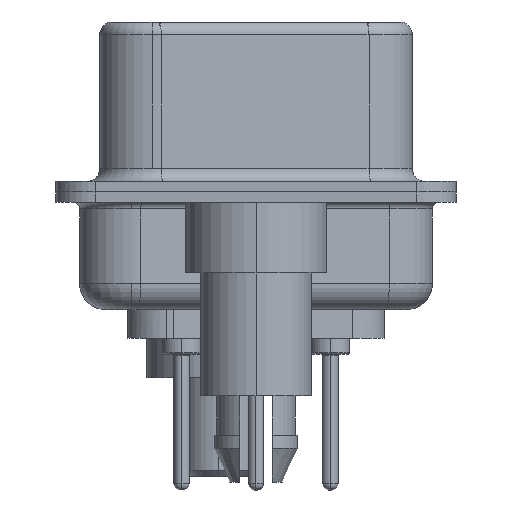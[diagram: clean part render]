
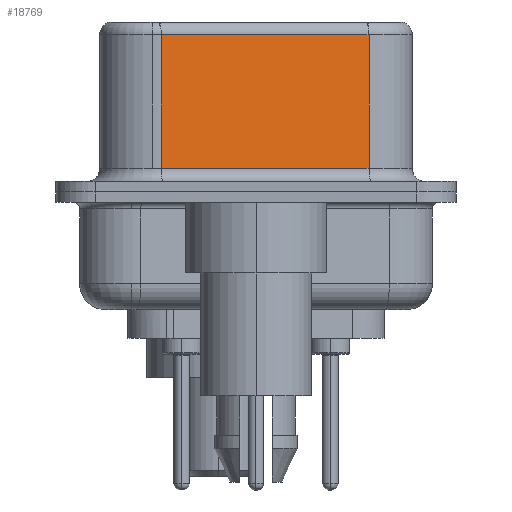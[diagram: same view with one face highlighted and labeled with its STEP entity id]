
A CAD part, left-side view. The second image highlights one B-rep face of the part: STEP entity #18769.
In plain terms, the highlighted planar face has unit normal (-0.985, -0.174, 0).
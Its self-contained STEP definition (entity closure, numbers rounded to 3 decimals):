
#282 = ORIENTED_EDGE ( 'NONE', *, *, #14902, .T. ) ;
#1563 = CARTESIAN_POINT ( 'NONE',  ( 3.73, 3.628, 6.02 ) ) ;
#2140 = VECTOR ( 'NONE', #11629, 1000. ) ;
#2462 = EDGE_CURVE ( 'NONE', #9417, #10179, #24107, .T. ) ;
#3331 = VERTEX_POINT ( 'NONE', #27265 ) ;
#6286 = ORIENTED_EDGE ( 'NONE', *, *, #25383, .T. ) ;
#7864 = CARTESIAN_POINT ( 'NONE',  ( 5.132, -4.322, 6.02 ) ) ;
#8260 = FACE_OUTER_BOUND ( 'NONE', #10070, .T. ) ;
#9417 = VERTEX_POINT ( 'NONE', #7864 ) ;
#9954 = CARTESIAN_POINT ( 'NONE',  ( 3.73, 3.628, 6.52 ) ) ;
#9983 = CARTESIAN_POINT ( 'NONE',  ( 5.132, -4.322, 6.02 ) ) ;
#10053 = CARTESIAN_POINT ( 'NONE',  ( 5.132, -4.322, 0.9 ) ) ;
#10059 = VERTEX_POINT ( 'NONE', #10053 ) ;
#10070 = EDGE_LOOP ( 'NONE', ( #21102, #13907, #282, #6286 ) ) ;
#10179 = VERTEX_POINT ( 'NONE', #1563 ) ;
#10293 = LINE ( 'NONE', #9954, #21693 ) ;
#11144 = DIRECTION ( 'NONE',  ( 0.985, 0.174, 0. ) ) ;
#11485 = CARTESIAN_POINT ( 'NONE',  ( 5.132, -4.322, 0.9 ) ) ;
#11629 = DIRECTION ( 'NONE',  ( 0., 0., -1. ) ) ;
#13636 = DIRECTION ( 'NONE',  ( 0.174, -0.985, 0. ) ) ;
#13907 = ORIENTED_EDGE ( 'NONE', *, *, #2462, .T. ) ;
#14902 = EDGE_CURVE ( 'NONE', #10179, #3331, #10293, .T. ) ;
#15679 = VECTOR ( 'NONE', #13636, 1000. ) ;
#16697 = DIRECTION ( 'NONE',  ( -0.174, 0.985, 0. ) ) ;
#17646 = AXIS2_PLACEMENT_3D ( 'NONE', #20118, #11144, #27052 ) ;
#18029 = VECTOR ( 'NONE', #16697, 1000. ) ;
#18769 = ADVANCED_FACE ( 'NONE', ( #8260 ), #20221, .F. ) ;
#19395 = LINE ( 'NONE', #25253, #2140 ) ;
#20118 = CARTESIAN_POINT ( 'NONE',  ( 5.132, -4.322, 6.52 ) ) ;
#20221 = PLANE ( 'NONE',  #17646 ) ;
#21102 = ORIENTED_EDGE ( 'NONE', *, *, #28424, .F. ) ;
#21693 = VECTOR ( 'NONE', #28230, 1000. ) ;
#24107 = LINE ( 'NONE', #9983, #18029 ) ;
#25253 = CARTESIAN_POINT ( 'NONE',  ( 5.132, -4.322, 6.52 ) ) ;
#25383 = EDGE_CURVE ( 'NONE', #3331, #10059, #28520, .T. ) ;
#27052 = DIRECTION ( 'NONE',  ( -0.174, 0.985, 0. ) ) ;
#27265 = CARTESIAN_POINT ( 'NONE',  ( 3.73, 3.628, 0.9 ) ) ;
#28230 = DIRECTION ( 'NONE',  ( 0., 0., -1. ) ) ;
#28424 = EDGE_CURVE ( 'NONE', #9417, #10059, #19395, .T. ) ;
#28520 = LINE ( 'NONE', #11485, #15679 ) ;
